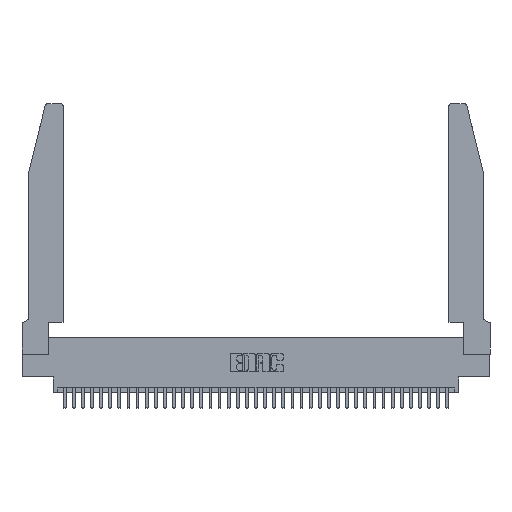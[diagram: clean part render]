
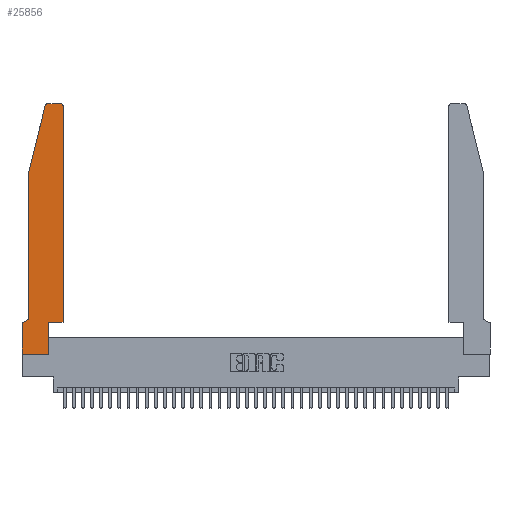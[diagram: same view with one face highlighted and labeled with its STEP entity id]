
A CAD part, top view. The second image highlights one B-rep face of the part: STEP entity #25856.
In plain terms, the highlighted planar face has unit normal (0, 0, 1).
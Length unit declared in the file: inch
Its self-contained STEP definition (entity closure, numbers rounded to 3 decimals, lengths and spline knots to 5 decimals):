
#92 = ORIENTED_EDGE ( 'NONE', *, *, #38418, .T. ) ;
#229 = CARTESIAN_POINT ( 'NONE',  ( 0.2865, 0.35, 0.37 ) ) ;
#1777 = CARTESIAN_POINT ( 'NONE',  ( 0.4505, 0.35, 0.37 ) ) ;
#2336 = CARTESIAN_POINT ( 'NONE',  ( 0.0055, 0.35, 0.37 ) ) ;
#2671 = AXIS2_PLACEMENT_3D ( 'NONE', #4294, #22232, #7277 ) ;
#3618 = VECTOR ( 'NONE', #33515, 39.37008 ) ;
#3672 = VERTEX_POINT ( 'NONE', #2336 ) ;
#4013 = ORIENTED_EDGE ( 'NONE', *, *, #11605, .T. ) ;
#4279 = LINE ( 'NONE', #229, #31772 ) ;
#4294 = CARTESIAN_POINT ( 'NONE',  ( 0., 0.35, 0.37 ) ) ;
#4348 = CIRCLE ( 'NONE', #10155, 0.03 ) ;
#4620 = VECTOR ( 'NONE', #29245, 39.37008 ) ;
#4795 = VERTEX_POINT ( 'NONE', #38471 ) ;
#5056 = CARTESIAN_POINT ( 'NONE',  ( 0.284, 2.75, 0.37 ) ) ;
#5063 = CARTESIAN_POINT ( 'NONE',  ( 0.25487, 2.72718, 0.37 ) ) ;
#5176 = VERTEX_POINT ( 'NONE', #12716 ) ;
#5492 = VECTOR ( 'NONE', #36263, 39.37008 ) ;
#7277 = DIRECTION ( 'NONE',  ( 1., 0., 0. ) ) ;
#8564 = CIRCLE ( 'NONE', #18773, 0.07 ) ;
#8718 = DIRECTION ( 'NONE',  ( 1., 0., 0. ) ) ;
#8817 = CARTESIAN_POINT ( 'NONE',  ( 0.284, 2.72, 0.37 ) ) ;
#8842 = CIRCLE ( 'NONE', #25533, 0.03 ) ;
#8945 = VECTOR ( 'NONE', #30067, 39.37008 ) ;
#9915 = CARTESIAN_POINT ( 'NONE',  ( 0., 0., 0.37 ) ) ;
#10155 = AXIS2_PLACEMENT_3D ( 'NONE', #37196, #13451, #37322 ) ;
#10238 = CARTESIAN_POINT ( 'NONE',  ( 0.4505, 0.35, 0.37 ) ) ;
#10663 = EDGE_CURVE ( 'NONE', #3672, #12700, #28892, .T. ) ;
#11534 = VECTOR ( 'NONE', #17119, 39.37008 ) ;
#11605 = EDGE_CURVE ( 'NONE', #13151, #26043, #8842, .T. ) ;
#12074 = CARTESIAN_POINT ( 'NONE',  ( 0.2865, 0., 0.37 ) ) ;
#12207 = DIRECTION ( 'NONE',  ( 0., 0., 1. ) ) ;
#12399 = CARTESIAN_POINT ( 'NONE',  ( 0.2605, 2.75, 0.37 ) ) ;
#12700 = VERTEX_POINT ( 'NONE', #35297 ) ;
#12716 = CARTESIAN_POINT ( 'NONE',  ( 0.4505, 2.72, 0.37 ) ) ;
#13013 = CARTESIAN_POINT ( 'NONE',  ( 0.0755, 0.42, 0.37 ) ) ;
#13151 = VERTEX_POINT ( 'NONE', #5056 ) ;
#13394 = ORIENTED_EDGE ( 'NONE', *, *, #28638, .T. ) ;
#13451 = DIRECTION ( 'NONE',  ( 0., 0., 1. ) ) ;
#13499 = VERTEX_POINT ( 'NONE', #24557 ) ;
#14166 = EDGE_CURVE ( 'NONE', #15479, #37333, #25343, .T. ) ;
#14596 = CARTESIAN_POINT ( 'NONE',  ( 0.4505, 0.35, 0.37 ) ) ;
#14655 = EDGE_CURVE ( 'NONE', #5176, #31276, #4348, .T. ) ;
#14777 = ORIENTED_EDGE ( 'NONE', *, *, #31556, .T. ) ;
#15479 = VERTEX_POINT ( 'NONE', #36228 ) ;
#17113 = DIRECTION ( 'NONE',  ( 0., 0., -1. ) ) ;
#17119 = DIRECTION ( 'NONE',  ( -0.239, -0.971, 0. ) ) ;
#17907 = ORIENTED_EDGE ( 'NONE', *, *, #38450, .T. ) ;
#18773 = AXIS2_PLACEMENT_3D ( 'NONE', #22805, #17113, #25687 ) ;
#20123 = ORIENTED_EDGE ( 'NONE', *, *, #21168, .T. ) ;
#20809 = VERTEX_POINT ( 'NONE', #12074 ) ;
#20859 = LINE ( 'NONE', #9915, #5492 ) ;
#21168 = EDGE_CURVE ( 'NONE', #37333, #3672, #8564, .T. ) ;
#22232 = DIRECTION ( 'NONE',  ( 0., 0., 1. ) ) ;
#22263 = ORIENTED_EDGE ( 'NONE', *, *, #14166, .T. ) ;
#22805 = CARTESIAN_POINT ( 'NONE',  ( 0.0055, 0.42, 0.37 ) ) ;
#23035 = VERTEX_POINT ( 'NONE', #1777 ) ;
#23645 = LINE ( 'NONE', #12399, #3618 ) ;
#23655 = DIRECTION ( 'NONE',  ( 0., -1., 0. ) ) ;
#24557 = CARTESIAN_POINT ( 'NONE',  ( 0., 0., 0.37 ) ) ;
#24751 = LINE ( 'NONE', #27296, #8945 ) ;
#25273 = ORIENTED_EDGE ( 'NONE', *, *, #10663, .T. ) ;
#25343 = LINE ( 'NONE', #26653, #35668 ) ;
#25533 = AXIS2_PLACEMENT_3D ( 'NONE', #8817, #12207, #29811 ) ;
#25687 = DIRECTION ( 'NONE',  ( -1., 0., 0. ) ) ;
#25856 = ADVANCED_FACE ( 'NONE', ( #28816 ), #34002, .T. ) ;
#26043 = VERTEX_POINT ( 'NONE', #5063 ) ;
#26653 = CARTESIAN_POINT ( 'NONE',  ( 0.0755, 2., 0.37 ) ) ;
#27296 = CARTESIAN_POINT ( 'NONE',  ( 0., 0., 0.37 ) ) ;
#27703 = LINE ( 'NONE', #10238, #36604 ) ;
#28638 = EDGE_CURVE ( 'NONE', #26043, #15479, #37181, .T. ) ;
#28816 = FACE_OUTER_BOUND ( 'NONE', #29722, .T. ) ;
#28892 = LINE ( 'NONE', #35529, #4620 ) ;
#29245 = DIRECTION ( 'NONE',  ( -1., 0., 0. ) ) ;
#29722 = EDGE_LOOP ( 'NONE', ( #17907, #4013, #13394, #22263, #20123, #25273, #92, #36383, #14777, #37607, #31397, #32678 ) ) ;
#29811 = DIRECTION ( 'NONE',  ( 1., 0., 0. ) ) ;
#29916 = EDGE_CURVE ( 'NONE', #23035, #5176, #27703, .T. ) ;
#30067 = DIRECTION ( 'NONE',  ( 1., 0., 0. ) ) ;
#31276 = VERTEX_POINT ( 'NONE', #31625 ) ;
#31397 = ORIENTED_EDGE ( 'NONE', *, *, #29916, .T. ) ;
#31527 = EDGE_CURVE ( 'NONE', #4795, #23035, #37875, .T. ) ;
#31556 = EDGE_CURVE ( 'NONE', #20809, #4795, #4279, .T. ) ;
#31625 = CARTESIAN_POINT ( 'NONE',  ( 0.4205, 2.75, 0.37 ) ) ;
#31772 = VECTOR ( 'NONE', #35836, 39.37008 ) ;
#32678 = ORIENTED_EDGE ( 'NONE', *, *, #14655, .T. ) ;
#32731 = EDGE_CURVE ( 'NONE', #13499, #20809, #24751, .T. ) ;
#33515 = DIRECTION ( 'NONE',  ( -1., 0., 0. ) ) ;
#34002 = PLANE ( 'NONE',  #2671 ) ;
#34223 = DIRECTION ( 'NONE',  ( 0., 1., 0. ) ) ;
#35297 = CARTESIAN_POINT ( 'NONE',  ( 0., 0.35, 0.37 ) ) ;
#35529 = CARTESIAN_POINT ( 'NONE',  ( 0.0755, 0.35, 0.37 ) ) ;
#35668 = VECTOR ( 'NONE', #23655, 39.37008 ) ;
#35836 = DIRECTION ( 'NONE',  ( 0., 1., 0. ) ) ;
#36228 = CARTESIAN_POINT ( 'NONE',  ( 0.0755, 2., 0.37 ) ) ;
#36263 = DIRECTION ( 'NONE',  ( 0., -1., 0. ) ) ;
#36383 = ORIENTED_EDGE ( 'NONE', *, *, #32731, .T. ) ;
#36604 = VECTOR ( 'NONE', #34223, 39.37008 ) ;
#37181 = LINE ( 'NONE', #38271, #11534 ) ;
#37196 = CARTESIAN_POINT ( 'NONE',  ( 0.4205, 2.72, 0.37 ) ) ;
#37322 = DIRECTION ( 'NONE',  ( 1., 0., 0. ) ) ;
#37333 = VERTEX_POINT ( 'NONE', #13013 ) ;
#37607 = ORIENTED_EDGE ( 'NONE', *, *, #31527, .T. ) ;
#37875 = LINE ( 'NONE', #14596, #38337 ) ;
#38271 = CARTESIAN_POINT ( 'NONE',  ( 0.0755, 2., 0.37 ) ) ;
#38337 = VECTOR ( 'NONE', #8718, 39.37008 ) ;
#38418 = EDGE_CURVE ( 'NONE', #12700, #13499, #20859, .T. ) ;
#38450 = EDGE_CURVE ( 'NONE', #31276, #13151, #23645, .T. ) ;
#38471 = CARTESIAN_POINT ( 'NONE',  ( 0.2865, 0.35, 0.37 ) ) ;
